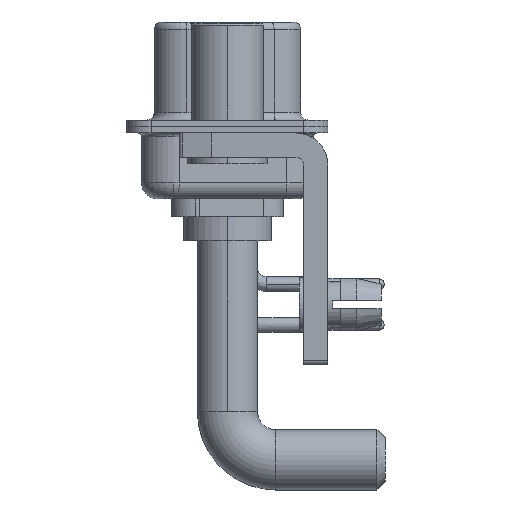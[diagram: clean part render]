
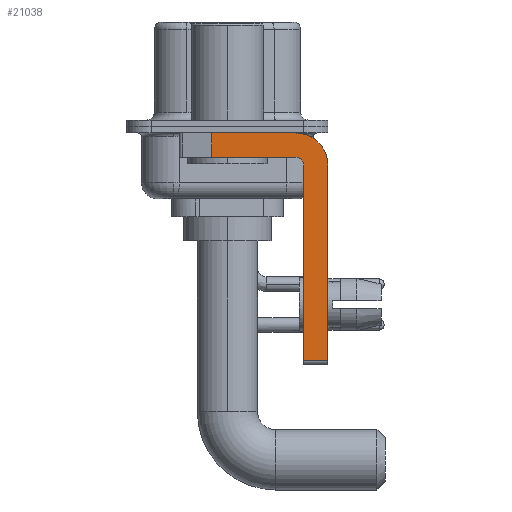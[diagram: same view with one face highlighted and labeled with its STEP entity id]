
A CAD part, left-side view. The second image highlights one B-rep face of the part: STEP entity #21038.
In plain terms, the highlighted planar face has unit normal (-1, 0, 0).
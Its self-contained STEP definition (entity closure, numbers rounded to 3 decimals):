
#249 = ORIENTED_EDGE ( 'NONE', *, *, #2576, .F. ) ;
#644 = EDGE_LOOP ( 'NONE', ( #23845, #26546, #12111, #22396, #8357, #10226, #249, #26975 ) ) ;
#1658 = AXIS2_PLACEMENT_3D ( 'NONE', #11374, #13679, #25930 ) ;
#1960 = VECTOR ( 'NONE', #11274, 1000. ) ;
#1999 = VECTOR ( 'NONE', #16480, 1000. ) ;
#2089 = DIRECTION ( 'NONE',  ( 1., 0., 0. ) ) ;
#2114 = CARTESIAN_POINT ( 'NONE',  ( -2.9, -6.25, -2.4 ) ) ;
#2576 = EDGE_CURVE ( 'NONE', #12191, #3854, #22498, .T. ) ;
#3582 = EDGE_CURVE ( 'NONE', #3970, #19696, #6000, .T. ) ;
#3854 = VERTEX_POINT ( 'NONE', #4914 ) ;
#3970 = VERTEX_POINT ( 'NONE', #29291 ) ;
#4371 = CARTESIAN_POINT ( 'NONE',  ( -2.9, -4.25, -2.4 ) ) ;
#4914 = CARTESIAN_POINT ( 'NONE',  ( -2.9, -6.25, -14.55 ) ) ;
#5387 = LINE ( 'NONE', #26252, #7997 ) ;
#6000 = LINE ( 'NONE', #22109, #13637 ) ;
#7223 = EDGE_CURVE ( 'NONE', #19863, #3854, #28421, .T. ) ;
#7946 = LINE ( 'NONE', #12257, #10797 ) ;
#7997 = VECTOR ( 'NONE', #28566, 1000. ) ;
#8269 = AXIS2_PLACEMENT_3D ( 'NONE', #4371, #2089, #13877 ) ;
#8357 = ORIENTED_EDGE ( 'NONE', *, *, #22260, .F. ) ;
#8992 = DIRECTION ( 'NONE',  ( 0., 0., -1. ) ) ;
#10226 = ORIENTED_EDGE ( 'NONE', *, *, #7223, .T. ) ;
#10240 = EDGE_CURVE ( 'NONE', #14165, #12191, #13396, .T. ) ;
#10797 = VECTOR ( 'NONE', #19590, 1000. ) ;
#11274 = DIRECTION ( 'NONE',  ( 0., 1., 0. ) ) ;
#11374 = CARTESIAN_POINT ( 'NONE',  ( -2.9, -4.25, -2.4 ) ) ;
#11926 = CIRCLE ( 'NONE', #17794, 0.5 ) ;
#12069 = CARTESIAN_POINT ( 'NONE',  ( -2.9, -4.25, -1.9 ) ) ;
#12111 = ORIENTED_EDGE ( 'NONE', *, *, #21176, .F. ) ;
#12191 = VERTEX_POINT ( 'NONE', #21058 ) ;
#12257 = CARTESIAN_POINT ( 'NONE',  ( -2.9, -4.75, -14.8 ) ) ;
#13396 = CIRCLE ( 'NONE', #1658, 2. ) ;
#13573 = CARTESIAN_POINT ( 'NONE',  ( -2.9, -4.75, -14.55 ) ) ;
#13627 = VERTEX_POINT ( 'NONE', #22877 ) ;
#13637 = VECTOR ( 'NONE', #24710, 1000. ) ;
#13679 = DIRECTION ( 'NONE',  ( 1., 0., 0. ) ) ;
#13877 = DIRECTION ( 'NONE',  ( 0., 0., -1. ) ) ;
#14165 = VERTEX_POINT ( 'NONE', #23594 ) ;
#14794 = DIRECTION ( 'NONE',  ( 0., 0., 1. ) ) ;
#16029 = CARTESIAN_POINT ( 'NONE',  ( -2.9, -4.25, -1.9 ) ) ;
#16480 = DIRECTION ( 'NONE',  ( 0., -1., 0. ) ) ;
#17700 = CARTESIAN_POINT ( 'NONE',  ( -2.9, 0.978, -1.9 ) ) ;
#17794 = AXIS2_PLACEMENT_3D ( 'NONE', #28765, #26448, #14794 ) ;
#19590 = DIRECTION ( 'NONE',  ( 0., 0., 1. ) ) ;
#19696 = VERTEX_POINT ( 'NONE', #17700 ) ;
#19704 = FACE_OUTER_BOUND ( 'NONE', #644, .T. ) ;
#19863 = VERTEX_POINT ( 'NONE', #13573 ) ;
#20919 = PLANE ( 'NONE',  #8269 ) ;
#21038 = ADVANCED_FACE ( 'NONE', ( #19704 ), #20919, .F. ) ;
#21058 = CARTESIAN_POINT ( 'NONE',  ( -2.9, -6.25, -2.4 ) ) ;
#21176 = EDGE_CURVE ( 'NONE', #28786, #19696, #22935, .T. ) ;
#22109 = CARTESIAN_POINT ( 'NONE',  ( -2.9, 0.978, -1.9 ) ) ;
#22260 = EDGE_CURVE ( 'NONE', #19863, #13627, #7946, .T. ) ;
#22396 = ORIENTED_EDGE ( 'NONE', *, *, #26629, .F. ) ;
#22498 = LINE ( 'NONE', #2114, #22908 ) ;
#22877 = CARTESIAN_POINT ( 'NONE',  ( -2.9, -4.75, -2.4 ) ) ;
#22908 = VECTOR ( 'NONE', #8992, 1000. ) ;
#22935 = LINE ( 'NONE', #16029, #1960 ) ;
#23594 = CARTESIAN_POINT ( 'NONE',  ( -2.9, -4.25, -0.4 ) ) ;
#23827 = CARTESIAN_POINT ( 'NONE',  ( -2.9, -4.25, -14.55 ) ) ;
#23845 = ORIENTED_EDGE ( 'NONE', *, *, #29568, .F. ) ;
#24710 = DIRECTION ( 'NONE',  ( 0., 0., -1. ) ) ;
#25930 = DIRECTION ( 'NONE',  ( 0., 0., -1. ) ) ;
#26252 = CARTESIAN_POINT ( 'NONE',  ( -2.9, 3., -0.4 ) ) ;
#26448 = DIRECTION ( 'NONE',  ( -1., 0., 0. ) ) ;
#26546 = ORIENTED_EDGE ( 'NONE', *, *, #3582, .T. ) ;
#26629 = EDGE_CURVE ( 'NONE', #13627, #28786, #11926, .T. ) ;
#26975 = ORIENTED_EDGE ( 'NONE', *, *, #10240, .F. ) ;
#28421 = LINE ( 'NONE', #23827, #1999 ) ;
#28566 = DIRECTION ( 'NONE',  ( 0., -1., 0. ) ) ;
#28765 = CARTESIAN_POINT ( 'NONE',  ( -2.9, -4.25, -2.4 ) ) ;
#28786 = VERTEX_POINT ( 'NONE', #12069 ) ;
#29291 = CARTESIAN_POINT ( 'NONE',  ( -2.9, 0.978, -0.4 ) ) ;
#29568 = EDGE_CURVE ( 'NONE', #3970, #14165, #5387, .T. ) ;
